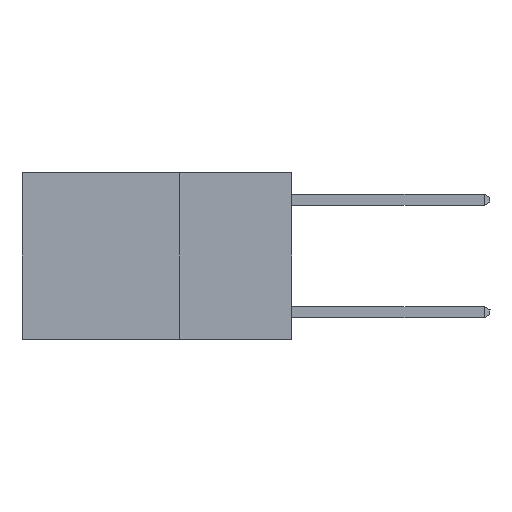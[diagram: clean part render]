
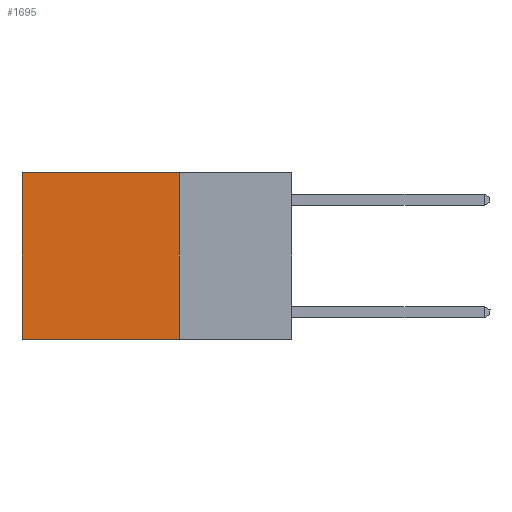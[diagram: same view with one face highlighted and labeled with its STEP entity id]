
A CAD part, left-side view. The second image highlights one B-rep face of the part: STEP entity #1695.
In plain terms, the highlighted planar face has unit normal (-1, 0, 0).
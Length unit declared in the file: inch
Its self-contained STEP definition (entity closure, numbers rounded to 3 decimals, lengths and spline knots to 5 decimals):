
#1695 = ADVANCED_FACE ( 'NONE', ( #6503 ), #15031, .F. ) ;
#2220 = EDGE_CURVE ( 'NONE', #10492, #24830, #15735, .T. ) ;
#3051 = DIRECTION ( 'NONE',  ( 0., 1., 0. ) ) ;
#3324 = CARTESIAN_POINT ( 'NONE',  ( 0.2625, 0.25, 0. ) ) ;
#4301 = EDGE_LOOP ( 'NONE', ( #21562, #6364, #5538, #16835 ) ) ;
#5538 = ORIENTED_EDGE ( 'NONE', *, *, #11482, .F. ) ;
#6364 = ORIENTED_EDGE ( 'NONE', *, *, #2220, .F. ) ;
#6462 = CARTESIAN_POINT ( 'NONE',  ( 0.2625, 0.6, -0.37 ) ) ;
#6503 = FACE_OUTER_BOUND ( 'NONE', #4301, .T. ) ;
#6819 = AXIS2_PLACEMENT_3D ( 'NONE', #14976, #14954, #14948 ) ;
#7584 = DIRECTION ( 'NONE',  ( 0., 1., 0. ) ) ;
#7669 = LINE ( 'NONE', #20584, #22399 ) ;
#7770 = CARTESIAN_POINT ( 'NONE',  ( 0.2625, 0.25, -0.37 ) ) ;
#8381 = VECTOR ( 'NONE', #3051, 39.37008 ) ;
#9595 = EDGE_CURVE ( 'NONE', #10457, #24830, #11511, .T. ) ;
#10012 = EDGE_CURVE ( 'NONE', #10110, #10457, #18130, .T. ) ;
#10110 = VERTEX_POINT ( 'NONE', #3324 ) ;
#10457 = VERTEX_POINT ( 'NONE', #23504 ) ;
#10492 = VERTEX_POINT ( 'NONE', #18131 ) ;
#10898 = VECTOR ( 'NONE', #13644, 39.37008 ) ;
#11022 = CARTESIAN_POINT ( 'NONE',  ( 0.2625, 0.25, 0. ) ) ;
#11482 = EDGE_CURVE ( 'NONE', #10110, #10492, #7669, .T. ) ;
#11511 = LINE ( 'NONE', #19312, #10898 ) ;
#13644 = DIRECTION ( 'NONE',  ( 0., 0., -1. ) ) ;
#14948 = DIRECTION ( 'NONE',  ( 0., 0., -1. ) ) ;
#14954 = DIRECTION ( 'NONE',  ( 1., 0., 0. ) ) ;
#14976 = CARTESIAN_POINT ( 'NONE',  ( 0.2625, 0.25, 0. ) ) ;
#15031 = PLANE ( 'NONE',  #6819 ) ;
#15735 = LINE ( 'NONE', #7770, #20123 ) ;
#16835 = ORIENTED_EDGE ( 'NONE', *, *, #10012, .T. ) ;
#16877 = DIRECTION ( 'NONE',  ( 0., 0., -1. ) ) ;
#18130 = LINE ( 'NONE', #11022, #8381 ) ;
#18131 = CARTESIAN_POINT ( 'NONE',  ( 0.2625, 0.25, -0.37 ) ) ;
#19312 = CARTESIAN_POINT ( 'NONE',  ( 0.2625, 0.6, 0. ) ) ;
#20123 = VECTOR ( 'NONE', #7584, 39.37008 ) ;
#20584 = CARTESIAN_POINT ( 'NONE',  ( 0.2625, 0.25, 0. ) ) ;
#21562 = ORIENTED_EDGE ( 'NONE', *, *, #9595, .T. ) ;
#22399 = VECTOR ( 'NONE', #16877, 39.37008 ) ;
#23504 = CARTESIAN_POINT ( 'NONE',  ( 0.2625, 0.6, 0. ) ) ;
#24830 = VERTEX_POINT ( 'NONE', #6462 ) ;
